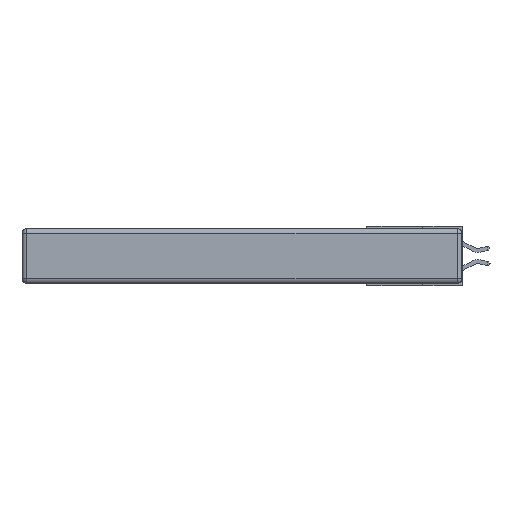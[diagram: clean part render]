
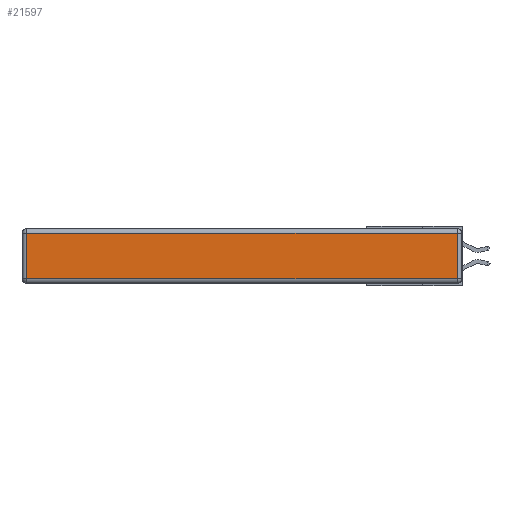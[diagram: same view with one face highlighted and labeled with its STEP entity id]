
A CAD part, left-side view. The second image highlights one B-rep face of the part: STEP entity #21597.
In plain terms, the highlighted planar face has unit normal (-1, 0, 0).
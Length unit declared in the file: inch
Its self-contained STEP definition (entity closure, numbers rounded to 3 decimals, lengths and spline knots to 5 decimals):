
#677 = CARTESIAN_POINT ( 'NONE',  ( 0., 2.72, -0.343 ) ) ;
#1281 = VECTOR ( 'NONE', #12568, 39.37008 ) ;
#1489 = VECTOR ( 'NONE', #17601, 39.37008 ) ;
#2097 = ORIENTED_EDGE ( 'NONE', *, *, #16489, .T. ) ;
#2533 = ORIENTED_EDGE ( 'NONE', *, *, #4606, .T. ) ;
#2894 = CARTESIAN_POINT ( 'NONE',  ( 0., 0.03, -0.343 ) ) ;
#3621 = DIRECTION ( 'NONE',  ( 0., 0., 1. ) ) ;
#4016 = AXIS2_PLACEMENT_3D ( 'NONE', #10985, #14517, #3621 ) ;
#4041 = FACE_OUTER_BOUND ( 'NONE', #22510, .T. ) ;
#4606 = EDGE_CURVE ( 'NONE', #23166, #7729, #15998, .T. ) ;
#6990 = ORIENTED_EDGE ( 'NONE', *, *, #18875, .T. ) ;
#7036 = VECTOR ( 'NONE', #13593, 39.37008 ) ;
#7314 = PLANE ( 'NONE',  #4016 ) ;
#7729 = VERTEX_POINT ( 'NONE', #12899 ) ;
#9707 = EDGE_CURVE ( 'NONE', #16483, #23566, #13362, .T. ) ;
#10985 = CARTESIAN_POINT ( 'NONE',  ( 0., 0., -0.343 ) ) ;
#11632 = ORIENTED_EDGE ( 'NONE', *, *, #9707, .T. ) ;
#12107 = DIRECTION ( 'NONE',  ( 0., 0., 1. ) ) ;
#12568 = DIRECTION ( 'NONE',  ( 0., -1., 0. ) ) ;
#12899 = CARTESIAN_POINT ( 'NONE',  ( 0., 0.03, -0.313 ) ) ;
#13362 = LINE ( 'NONE', #17677, #1489 ) ;
#13593 = DIRECTION ( 'NONE',  ( 0., 0., -1. ) ) ;
#14517 = DIRECTION ( 'NONE',  ( -1., 0., 0. ) ) ;
#15998 = LINE ( 'NONE', #23473, #1281 ) ;
#16483 = VERTEX_POINT ( 'NONE', #23169 ) ;
#16489 = EDGE_CURVE ( 'NONE', #7729, #16483, #23689, .T. ) ;
#17336 = VECTOR ( 'NONE', #12107, 39.37008 ) ;
#17601 = DIRECTION ( 'NONE',  ( 0., 1., 0. ) ) ;
#17677 = CARTESIAN_POINT ( 'NONE',  ( 0., 2.75, -0.03 ) ) ;
#18875 = EDGE_CURVE ( 'NONE', #23566, #23166, #23214, .T. ) ;
#20050 = CARTESIAN_POINT ( 'NONE',  ( 0., 2.72, -0.03 ) ) ;
#20900 = CARTESIAN_POINT ( 'NONE',  ( 0., 2.72, -0.313 ) ) ;
#21597 = ADVANCED_FACE ( 'NONE', ( #4041 ), #7314, .T. ) ;
#22510 = EDGE_LOOP ( 'NONE', ( #2533, #2097, #11632, #6990 ) ) ;
#23166 = VERTEX_POINT ( 'NONE', #20900 ) ;
#23169 = CARTESIAN_POINT ( 'NONE',  ( 0., 0.03, -0.03 ) ) ;
#23214 = LINE ( 'NONE', #677, #7036 ) ;
#23473 = CARTESIAN_POINT ( 'NONE',  ( 0., 0., -0.313 ) ) ;
#23566 = VERTEX_POINT ( 'NONE', #20050 ) ;
#23689 = LINE ( 'NONE', #2894, #17336 ) ;
